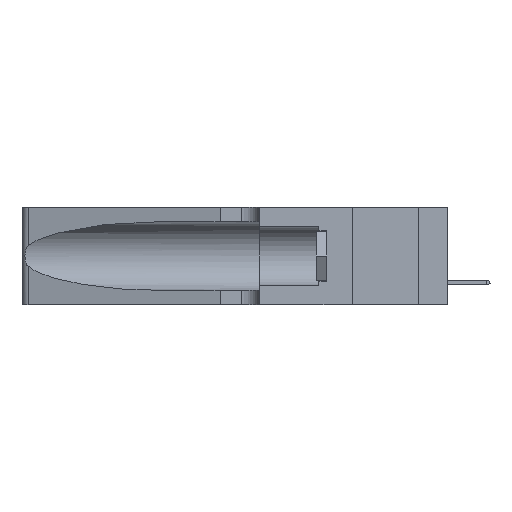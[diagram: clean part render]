
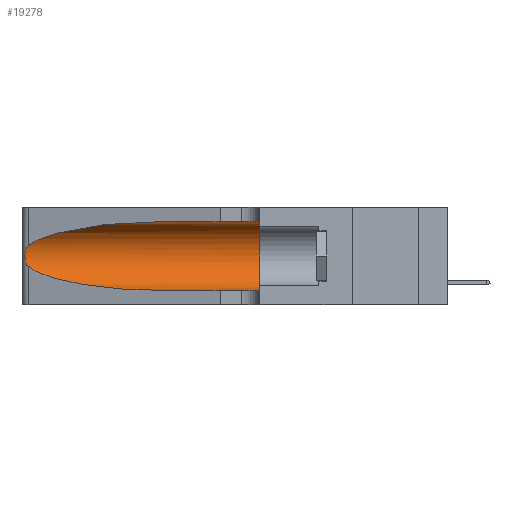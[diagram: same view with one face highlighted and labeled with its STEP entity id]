
A CAD part, left-side view. The second image highlights one B-rep face of the part: STEP entity #19278.
In plain terms, the highlighted cylindrical face has radius 3.308 mm (diameter 6.617 mm), a partial arc.
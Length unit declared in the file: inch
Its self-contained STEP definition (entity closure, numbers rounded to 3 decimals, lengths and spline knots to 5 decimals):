
#213 = DIRECTION ( 'NONE',  ( 0., 0., 1. ) ) ;
#789 = CARTESIAN_POINT ( 'NONE',  ( 0.25487, 1.22718, 0.14631 ) ) ;
#1739 =( BOUNDED_CURVE ( )  B_SPLINE_CURVE ( 3, ( #14881, #5795, #3460, #17268 ),
 .UNSPECIFIED., .F., .F. ) 
 B_SPLINE_CURVE_WITH_KNOTS ( ( 4, 4 ),
 ( 1.5708, 2.84003 ),
 .UNSPECIFIED. ) 
 CURVE ( )  GEOMETRIC_REPRESENTATION_ITEM ( )  RATIONAL_B_SPLINE_CURVE ( ( 1., 0.87, 0.87, 1. ) ) 
 REPRESENTATION_ITEM ( '' )  );
#2255 = DIRECTION ( 'NONE',  ( 0., -1., 0. ) ) ;
#2429 = EDGE_LOOP ( 'NONE', ( #15881, #21875, #28565, #26476, #7361, #12543 ) ) ;
#2685 = LINE ( 'NONE', #15570, #22833 ) ;
#2848 = DIRECTION ( 'NONE',  ( 0., -1., 0. ) ) ;
#2904 = DIRECTION ( 'NONE',  ( 0., 0., -1. ) ) ;
#3056 = CARTESIAN_POINT ( 'NONE',  ( 0.25487, 1.22718, 0.14631 ) ) ;
#3073 = VERTEX_POINT ( 'NONE', #22074 ) ;
#3134 = CARTESIAN_POINT ( 'NONE',  ( 0.25487, 1.22718, 0.22369 ) ) ;
#3277 = CARTESIAN_POINT ( 'NONE',  ( 0.2373, 1.15595, 0.08982 ) ) ;
#3460 = CARTESIAN_POINT ( 'NONE',  ( 0.2373, 1.15595, 0.28018 ) ) ;
#3508 = CARTESIAN_POINT ( 'NONE',  ( 0.1305, 0.72297, 0.05475 ) ) ;
#5226 = CARTESIAN_POINT ( 'NONE',  ( 0.25555, 1.22993, 0.14849 ) ) ;
#5795 = CARTESIAN_POINT ( 'NONE',  ( 0.18966, 0.96281, 0.31525 ) ) ;
#6281 = CARTESIAN_POINT ( 'NONE',  ( 0.1305, 0.72297, 0.05475 ) ) ;
#6936 = CARTESIAN_POINT ( 'NONE',  ( 0.25555, 1.22994, 0.2215 ) ) ;
#7264 = CARTESIAN_POINT ( 'NONE',  ( 0.26018, 1.23835, 0.19895 ) ) ;
#7361 = ORIENTED_EDGE ( 'NONE', *, *, #22229, .F. ) ;
#7775 = AXIS2_PLACEMENT_3D ( 'NONE', #17396, #27084, #2904 ) ;
#8919 = CARTESIAN_POINT ( 'NONE',  ( 0.1305, 0.72297, 0.31525 ) ) ;
#10111 = CARTESIAN_POINT ( 'NONE',  ( 0.25854, 1.2359, 0.20912 ) ) ;
#10876 = VERTEX_POINT ( 'NONE', #8919 ) ;
#10968 = AXIS2_PLACEMENT_3D ( 'NONE', #14534, #30054, #213 ) ;
#12336 = CARTESIAN_POINT ( 'NONE',  ( 0.26075, 1.23896, 0.19203 ) ) ;
#12455 = B_SPLINE_CURVE_WITH_KNOTS ( 'NONE', 3,
 ( #27014, #6936, #27655, #32749, #10111, #7264, #12336, #29984, #17432, #20673, #20349, #23099, #5226, #12863 ),
 .UNSPECIFIED., .F., .F.,
 ( 4, 2, 2, 2, 2, 2, 4 ),
 ( 0., 0.00027, 0.00053, 0.00107, 0.0016, 0.00187, 0.00214 ),
 .UNSPECIFIED. ) ;
#12475 = CIRCLE ( 'NONE', #10968, 0.13025 ) ;
#12543 = ORIENTED_EDGE ( 'NONE', *, *, #13521, .F. ) ;
#12863 = CARTESIAN_POINT ( 'NONE',  ( 0.25487, 1.22718, 0.14631 ) ) ;
#13521 = EDGE_CURVE ( 'NONE', #10876, #27391, #24762, .T. ) ;
#14534 = CARTESIAN_POINT ( 'NONE',  ( 0.1305, 0.35, 0.185 ) ) ;
#14881 = CARTESIAN_POINT ( 'NONE',  ( 0.1305, 0.72297, 0.31525 ) ) ;
#15570 = CARTESIAN_POINT ( 'NONE',  ( 0.1305, 1.61858, 0.05475 ) ) ;
#15881 = ORIENTED_EDGE ( 'NONE', *, *, #20154, .T. ) ;
#17268 = CARTESIAN_POINT ( 'NONE',  ( 0.25487, 1.22718, 0.22369 ) ) ;
#17396 = CARTESIAN_POINT ( 'NONE',  ( 0.1305, 1.61858, 0.185 ) ) ;
#17432 = CARTESIAN_POINT ( 'NONE',  ( 0.26017, 1.23833, 0.17102 ) ) ;
#19278 = ADVANCED_FACE ( 'NONE', ( #29487 ), #22330, .F. ) ;
#20154 = EDGE_CURVE ( 'NONE', #10876, #21330, #1739, .T. ) ;
#20349 = CARTESIAN_POINT ( 'NONE',  ( 0.25789, 1.23486, 0.15765 ) ) ;
#20479 = EDGE_CURVE ( 'NONE', #32164, #3073, #2685, .T. ) ;
#20673 = CARTESIAN_POINT ( 'NONE',  ( 0.25856, 1.23593, 0.16098 ) ) ;
#21330 = VERTEX_POINT ( 'NONE', #3134 ) ;
#21545 = VERTEX_POINT ( 'NONE', #789 ) ;
#21875 = ORIENTED_EDGE ( 'NONE', *, *, #29729, .T. ) ;
#22074 = CARTESIAN_POINT ( 'NONE',  ( 0.1305, 0.35, 0.05475 ) ) ;
#22229 = EDGE_CURVE ( 'NONE', #27391, #3073, #12475, .T. ) ;
#22330 = CYLINDRICAL_SURFACE ( 'NONE', #7775, 0.13025 ) ;
#22833 = VECTOR ( 'NONE', #2848, 39.37008 ) ;
#23099 = CARTESIAN_POINT ( 'NONE',  ( 0.25639, 1.23186, 0.15144 ) ) ;
#23482 = CARTESIAN_POINT ( 'NONE',  ( 0.18966, 0.96281, 0.05475 ) ) ;
#24762 = LINE ( 'NONE', #32504, #29536 ) ;
#26174 = EDGE_CURVE ( 'NONE', #21545, #32164, #31508, .T. ) ;
#26476 = ORIENTED_EDGE ( 'NONE', *, *, #20479, .T. ) ;
#27014 = CARTESIAN_POINT ( 'NONE',  ( 0.25487, 1.22718, 0.22369 ) ) ;
#27084 = DIRECTION ( 'NONE',  ( 0., -1., 0. ) ) ;
#27391 = VERTEX_POINT ( 'NONE', #32165 ) ;
#27655 = CARTESIAN_POINT ( 'NONE',  ( 0.25639, 1.23184, 0.21858 ) ) ;
#28565 = ORIENTED_EDGE ( 'NONE', *, *, #26174, .T. ) ;
#29487 = FACE_OUTER_BOUND ( 'NONE', #2429, .T. ) ;
#29536 = VECTOR ( 'NONE', #2255, 39.37008 ) ;
#29729 = EDGE_CURVE ( 'NONE', #21330, #21545, #12455, .T. ) ;
#29984 = CARTESIAN_POINT ( 'NONE',  ( 0.26075, 1.23896, 0.178 ) ) ;
#30054 = DIRECTION ( 'NONE',  ( 0., 1., 0. ) ) ;
#31508 =( BOUNDED_CURVE ( )  B_SPLINE_CURVE ( 3, ( #3056, #3277, #23482, #3508 ),
 .UNSPECIFIED., .F., .T. ) 
 B_SPLINE_CURVE_WITH_KNOTS ( ( 4, 4 ),
 ( 3.44316, 4.71239 ),
 .UNSPECIFIED. ) 
 CURVE ( )  GEOMETRIC_REPRESENTATION_ITEM ( )  RATIONAL_B_SPLINE_CURVE ( ( 1., 0.87, 0.87, 1. ) ) 
 REPRESENTATION_ITEM ( '' )  );
#32164 = VERTEX_POINT ( 'NONE', #6281 ) ;
#32165 = CARTESIAN_POINT ( 'NONE',  ( 0.1305, 0.35, 0.31525 ) ) ;
#32504 = CARTESIAN_POINT ( 'NONE',  ( 0.1305, 1.61858, 0.31525 ) ) ;
#32749 = CARTESIAN_POINT ( 'NONE',  ( 0.25787, 1.23484, 0.2124 ) ) ;
